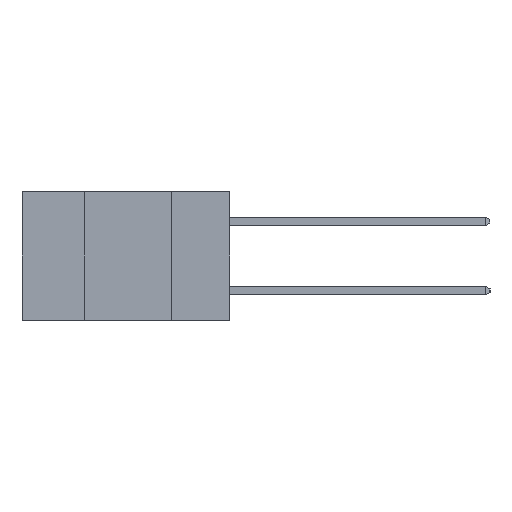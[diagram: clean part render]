
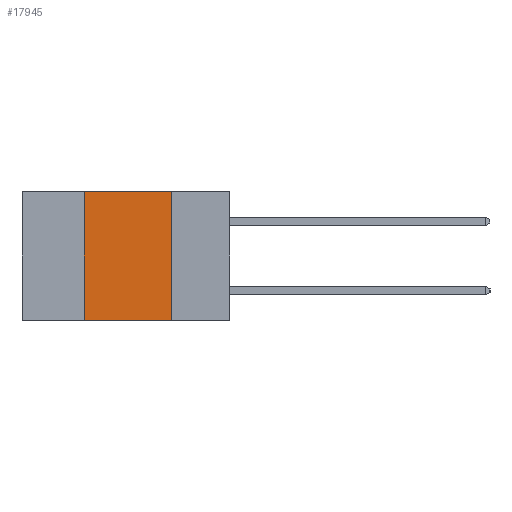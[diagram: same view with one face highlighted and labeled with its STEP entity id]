
A CAD part, left-side view. The second image highlights one B-rep face of the part: STEP entity #17945.
In plain terms, the highlighted planar face has unit normal (-1, 0, 0).
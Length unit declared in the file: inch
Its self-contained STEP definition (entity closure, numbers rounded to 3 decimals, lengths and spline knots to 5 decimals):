
#162 = EDGE_CURVE ( 'NONE', #22851, #18875, #14880, .T. ) ;
#817 = VECTOR ( 'NONE', #6486, 39.37008 ) ;
#836 = CARTESIAN_POINT ( 'NONE',  ( 0., 0.42, -0.37 ) ) ;
#1522 = LINE ( 'NONE', #22229, #11580 ) ;
#1586 = ORIENTED_EDGE ( 'NONE', *, *, #162, .F. ) ;
#1816 = AXIS2_PLACEMENT_3D ( 'NONE', #18203, #10320, #24081 ) ;
#2872 = FACE_OUTER_BOUND ( 'NONE', #17778, .T. ) ;
#4982 = DIRECTION ( 'NONE',  ( 0., -1., 0. ) ) ;
#5634 = ORIENTED_EDGE ( 'NONE', *, *, #6857, .F. ) ;
#6486 = DIRECTION ( 'NONE',  ( 0., -1., 0. ) ) ;
#6588 = VERTEX_POINT ( 'NONE', #13871 ) ;
#6857 = EDGE_CURVE ( 'NONE', #18875, #6588, #12115, .T. ) ;
#8141 = CARTESIAN_POINT ( 'NONE',  ( 0., 0.17, -0.37 ) ) ;
#10320 = DIRECTION ( 'NONE',  ( 1., 0., 0. ) ) ;
#11580 = VECTOR ( 'NONE', #14435, 39.37008 ) ;
#12115 = LINE ( 'NONE', #12559, #817 ) ;
#12244 = PLANE ( 'NONE',  #1816 ) ;
#12250 = EDGE_CURVE ( 'NONE', #22851, #14995, #12401, .T. ) ;
#12401 = LINE ( 'NONE', #12947, #22224 ) ;
#12559 = CARTESIAN_POINT ( 'NONE',  ( 0., 0.6, 0. ) ) ;
#12947 = CARTESIAN_POINT ( 'NONE',  ( 0., 0.6, -0.37 ) ) ;
#12981 = CARTESIAN_POINT ( 'NONE',  ( 0., 0.42, 0. ) ) ;
#13871 = CARTESIAN_POINT ( 'NONE',  ( 0., 0.17, 0. ) ) ;
#14435 = DIRECTION ( 'NONE',  ( 0., 0., -1. ) ) ;
#14880 = LINE ( 'NONE', #22365, #20085 ) ;
#14995 = VERTEX_POINT ( 'NONE', #8141 ) ;
#16294 = ORIENTED_EDGE ( 'NONE', *, *, #12250, .T. ) ;
#17778 = EDGE_LOOP ( 'NONE', ( #24216, #5634, #1586, #16294 ) ) ;
#17945 = ADVANCED_FACE ( 'NONE', ( #2872 ), #12244, .F. ) ;
#18203 = CARTESIAN_POINT ( 'NONE',  ( 0., 0.6, 0. ) ) ;
#18875 = VERTEX_POINT ( 'NONE', #12981 ) ;
#19339 = EDGE_CURVE ( 'NONE', #6588, #14995, #1522, .T. ) ;
#20085 = VECTOR ( 'NONE', #24012, 39.37008 ) ;
#22224 = VECTOR ( 'NONE', #4982, 39.37008 ) ;
#22229 = CARTESIAN_POINT ( 'NONE',  ( 0., 0.17, -0.37 ) ) ;
#22365 = CARTESIAN_POINT ( 'NONE',  ( 0., 0.42, -0.37 ) ) ;
#22851 = VERTEX_POINT ( 'NONE', #836 ) ;
#24012 = DIRECTION ( 'NONE',  ( 0., 0., 1. ) ) ;
#24081 = DIRECTION ( 'NONE',  ( 0., 0., -1. ) ) ;
#24216 = ORIENTED_EDGE ( 'NONE', *, *, #19339, .F. ) ;
